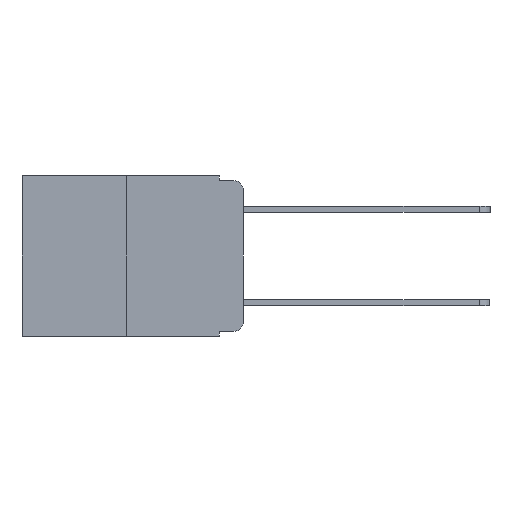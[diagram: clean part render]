
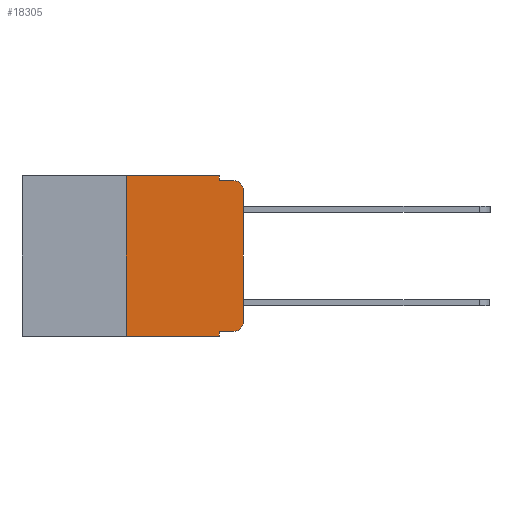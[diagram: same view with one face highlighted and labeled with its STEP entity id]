
A CAD part, left-side view. The second image highlights one B-rep face of the part: STEP entity #18305.
In plain terms, the highlighted planar face has unit normal (-1, 0, 0).
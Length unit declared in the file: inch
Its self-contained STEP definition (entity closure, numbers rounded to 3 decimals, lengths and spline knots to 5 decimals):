
#88 = ORIENTED_EDGE ( 'NONE', *, *, #2145, .T. ) ;
#291 = CARTESIAN_POINT ( 'NONE',  ( 0., 0.02, -0.03 ) ) ;
#297 = CARTESIAN_POINT ( 'NONE',  ( 0., 0.051, -0.343 ) ) ;
#644 = VECTOR ( 'NONE', #3420, 39.37008 ) ;
#696 = CARTESIAN_POINT ( 'NONE',  ( 0., 0.051, 0. ) ) ;
#748 = EDGE_CURVE ( 'NONE', #5425, #15150, #5211, .T. ) ;
#1669 = ORIENTED_EDGE ( 'NONE', *, *, #7935, .T. ) ;
#1869 = ORIENTED_EDGE ( 'NONE', *, *, #10897, .F. ) ;
#1976 = EDGE_CURVE ( 'NONE', #19134, #19321, #4357, .T. ) ;
#1984 = DIRECTION ( 'NONE',  ( 0., 0., -1. ) ) ;
#2145 = EDGE_CURVE ( 'NONE', #9497, #16834, #5156, .T. ) ;
#2335 = DIRECTION ( 'NONE',  ( 0., 0., -1. ) ) ;
#2751 = LINE ( 'NONE', #8588, #19971 ) ;
#2783 = CARTESIAN_POINT ( 'NONE',  ( 0., 0.051, 0. ) ) ;
#3117 = DIRECTION ( 'NONE',  ( 0., 0., -1. ) ) ;
#3420 = DIRECTION ( 'NONE',  ( 0., 0., -1. ) ) ;
#3818 = VECTOR ( 'NONE', #15648, 39.37008 ) ;
#3839 = CIRCLE ( 'NONE', #8333, 0.02 ) ;
#3968 = ORIENTED_EDGE ( 'NONE', *, *, #10135, .F. ) ;
#4216 = DIRECTION ( 'NONE',  ( 0., 0., 1. ) ) ;
#4357 = LINE ( 'NONE', #696, #16597 ) ;
#4704 = AXIS2_PLACEMENT_3D ( 'NONE', #10820, #12460, #2335 ) ;
#4781 = LINE ( 'NONE', #20298, #8212 ) ;
#5156 = CIRCLE ( 'NONE', #8675, 0.02 ) ;
#5211 = LINE ( 'NONE', #2783, #644 ) ;
#5344 = DIRECTION ( 'NONE',  ( 0., -1., 0. ) ) ;
#5379 = VERTEX_POINT ( 'NONE', #20833 ) ;
#5425 = VERTEX_POINT ( 'NONE', #12189 ) ;
#5451 = DIRECTION ( 'NONE',  ( 0., 0., 1. ) ) ;
#5655 = CARTESIAN_POINT ( 'NONE',  ( 0., 0.051, -0.01 ) ) ;
#6001 = LINE ( 'NONE', #15777, #18695 ) ;
#6510 = ORIENTED_EDGE ( 'NONE', *, *, #11883, .T. ) ;
#6963 = ORIENTED_EDGE ( 'NONE', *, *, #10472, .T. ) ;
#7935 = EDGE_CURVE ( 'NONE', #16918, #15150, #2751, .T. ) ;
#8212 = VECTOR ( 'NONE', #5451, 39.37008 ) ;
#8333 = AXIS2_PLACEMENT_3D ( 'NONE', #291, #12135, #1984 ) ;
#8356 = LINE ( 'NONE', #5655, #3818 ) ;
#8588 = CARTESIAN_POINT ( 'NONE',  ( 0., 0.473, -0.343 ) ) ;
#8675 = AXIS2_PLACEMENT_3D ( 'NONE', #16199, #14831, #3117 ) ;
#9232 = VECTOR ( 'NONE', #4216, 39.37008 ) ;
#9261 = CARTESIAN_POINT ( 'NONE',  ( 0., 0., 0. ) ) ;
#9497 = VERTEX_POINT ( 'NONE', #11013 ) ;
#9561 = DIRECTION ( 'NONE',  ( 0., 0., -1. ) ) ;
#9692 = CARTESIAN_POINT ( 'NONE',  ( 0., 0.051, 0. ) ) ;
#10109 = CARTESIAN_POINT ( 'NONE',  ( 0., 0.25, 0. ) ) ;
#10135 = EDGE_CURVE ( 'NONE', #10367, #19134, #6001, .T. ) ;
#10293 = CARTESIAN_POINT ( 'NONE',  ( 0., 0., -0.313 ) ) ;
#10367 = VERTEX_POINT ( 'NONE', #10109 ) ;
#10472 = EDGE_CURVE ( 'NONE', #13175, #5379, #3839, .T. ) ;
#10505 = CARTESIAN_POINT ( 'NONE',  ( 0., 0.25, -0.343 ) ) ;
#10626 = ORIENTED_EDGE ( 'NONE', *, *, #18187, .F. ) ;
#10820 = CARTESIAN_POINT ( 'NONE',  ( 0., 0.473, 0. ) ) ;
#10897 = EDGE_CURVE ( 'NONE', #19321, #5379, #8356, .T. ) ;
#11013 = CARTESIAN_POINT ( 'NONE',  ( 0., 0.02, -0.333 ) ) ;
#11097 = ORIENTED_EDGE ( 'NONE', *, *, #19715, .T. ) ;
#11194 = LINE ( 'NONE', #13522, #19917 ) ;
#11750 = ORIENTED_EDGE ( 'NONE', *, *, #748, .F. ) ;
#11883 = EDGE_CURVE ( 'NONE', #5425, #9497, #11194, .T. ) ;
#12135 = DIRECTION ( 'NONE',  ( -1., 0., 0. ) ) ;
#12189 = CARTESIAN_POINT ( 'NONE',  ( 0., 0.051, -0.333 ) ) ;
#12460 = DIRECTION ( 'NONE',  ( 1., 0., 0. ) ) ;
#13175 = VERTEX_POINT ( 'NONE', #13611 ) ;
#13522 = CARTESIAN_POINT ( 'NONE',  ( 0., 0.051, -0.333 ) ) ;
#13597 = LINE ( 'NONE', #9261, #9232 ) ;
#13611 = CARTESIAN_POINT ( 'NONE',  ( 0., 0., -0.03 ) ) ;
#14399 = FACE_OUTER_BOUND ( 'NONE', #16414, .T. ) ;
#14831 = DIRECTION ( 'NONE',  ( -1., 0., 0. ) ) ;
#15150 = VERTEX_POINT ( 'NONE', #297 ) ;
#15648 = DIRECTION ( 'NONE',  ( 0., -1., 0. ) ) ;
#15777 = CARTESIAN_POINT ( 'NONE',  ( 0., 0.473, 0. ) ) ;
#15811 = ORIENTED_EDGE ( 'NONE', *, *, #1976, .F. ) ;
#16199 = CARTESIAN_POINT ( 'NONE',  ( 0., 0.02, -0.313 ) ) ;
#16414 = EDGE_LOOP ( 'NONE', ( #11097, #6963, #1869, #15811, #3968, #10626, #1669, #11750, #6510, #88 ) ) ;
#16597 = VECTOR ( 'NONE', #9561, 39.37008 ) ;
#16834 = VERTEX_POINT ( 'NONE', #10293 ) ;
#16918 = VERTEX_POINT ( 'NONE', #10505 ) ;
#17428 = DIRECTION ( 'NONE',  ( 0., -1., 0. ) ) ;
#18054 = CARTESIAN_POINT ( 'NONE',  ( 0., 0.051, -0.01 ) ) ;
#18187 = EDGE_CURVE ( 'NONE', #16918, #10367, #4781, .T. ) ;
#18305 = ADVANCED_FACE ( 'NONE', ( #14399 ), #20645, .F. ) ;
#18695 = VECTOR ( 'NONE', #17428, 39.37008 ) ;
#19134 = VERTEX_POINT ( 'NONE', #9692 ) ;
#19321 = VERTEX_POINT ( 'NONE', #18054 ) ;
#19715 = EDGE_CURVE ( 'NONE', #16834, #13175, #13597, .T. ) ;
#19917 = VECTOR ( 'NONE', #20078, 39.37008 ) ;
#19971 = VECTOR ( 'NONE', #5344, 39.37008 ) ;
#20078 = DIRECTION ( 'NONE',  ( 0., -1., 0. ) ) ;
#20298 = CARTESIAN_POINT ( 'NONE',  ( 0., 0.25, 0. ) ) ;
#20645 = PLANE ( 'NONE',  #4704 ) ;
#20833 = CARTESIAN_POINT ( 'NONE',  ( 0., 0.02, -0.01 ) ) ;
